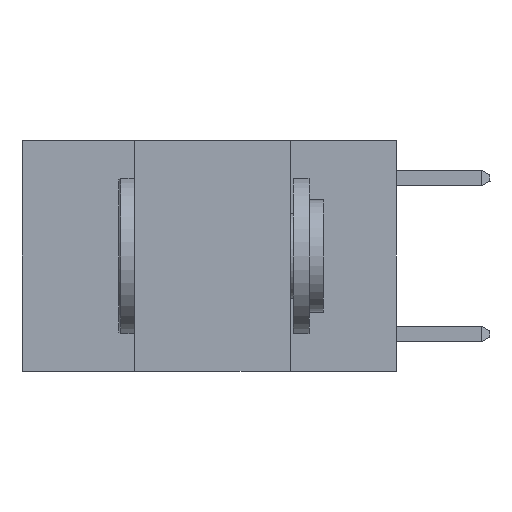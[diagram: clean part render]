
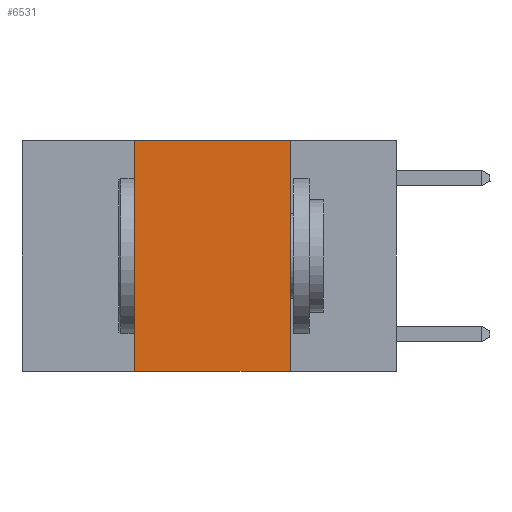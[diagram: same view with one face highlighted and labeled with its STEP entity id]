
A CAD part, left-side view. The second image highlights one B-rep face of the part: STEP entity #6531.
In plain terms, the highlighted planar face has unit normal (-1, 0, 0).
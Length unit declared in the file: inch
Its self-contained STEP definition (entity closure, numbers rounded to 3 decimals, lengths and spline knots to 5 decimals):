
#1452 = LINE ( 'NONE', #12778, #8683 ) ;
#1490 = LINE ( 'NONE', #7999, #16613 ) ;
#2187 = LINE ( 'NONE', #18214, #9373 ) ;
#4486 = EDGE_CURVE ( 'NONE', #6804, #16520, #1452, .T. ) ;
#4678 = VECTOR ( 'NONE', #15822, 39.37008 ) ;
#6480 = FACE_OUTER_BOUND ( 'NONE', #9676, .T. ) ;
#6512 = CARTESIAN_POINT ( 'NONE',  ( 0., 0.42, -0.37 ) ) ;
#6531 = ADVANCED_FACE ( 'NONE', ( #6480 ), #7337, .F. ) ;
#6561 = DIRECTION ( 'NONE',  ( 0., -1., 0. ) ) ;
#6804 = VERTEX_POINT ( 'NONE', #6512 ) ;
#7207 = ORIENTED_EDGE ( 'NONE', *, *, #15661, .F. ) ;
#7337 = PLANE ( 'NONE',  #16276 ) ;
#7359 = CARTESIAN_POINT ( 'NONE',  ( 0., 0.42, 0. ) ) ;
#7409 = ORIENTED_EDGE ( 'NONE', *, *, #14850, .F. ) ;
#7429 = ORIENTED_EDGE ( 'NONE', *, *, #16599, .F. ) ;
#7681 = ORIENTED_EDGE ( 'NONE', *, *, #4486, .T. ) ;
#7999 = CARTESIAN_POINT ( 'NONE',  ( 0., 0.6, 0. ) ) ;
#8031 = LINE ( 'NONE', #7359, #4678 ) ;
#8585 = DIRECTION ( 'NONE',  ( 0., 0., -1. ) ) ;
#8683 = VECTOR ( 'NONE', #15579, 39.37008 ) ;
#8747 = DIRECTION ( 'NONE',  ( 0., 0., -1. ) ) ;
#8867 = VERTEX_POINT ( 'NONE', #14411 ) ;
#9373 = VECTOR ( 'NONE', #8585, 39.37008 ) ;
#9676 = EDGE_LOOP ( 'NONE', ( #7207, #7409, #7429, #7681 ) ) ;
#10503 = CARTESIAN_POINT ( 'NONE',  ( 0., 0.17, -0.37 ) ) ;
#12778 = CARTESIAN_POINT ( 'NONE',  ( 0., 0.6, -0.37 ) ) ;
#13037 = CARTESIAN_POINT ( 'NONE',  ( 0., 0.6, 0. ) ) ;
#14411 = CARTESIAN_POINT ( 'NONE',  ( 0., 0.17, 0. ) ) ;
#14850 = EDGE_CURVE ( 'NONE', #17914, #8867, #1490, .T. ) ;
#15579 = DIRECTION ( 'NONE',  ( 0., -1., 0. ) ) ;
#15661 = EDGE_CURVE ( 'NONE', #8867, #16520, #2187, .T. ) ;
#15822 = DIRECTION ( 'NONE',  ( 0., 0., 1. ) ) ;
#16276 = AXIS2_PLACEMENT_3D ( 'NONE', #13037, #17110, #8747 ) ;
#16520 = VERTEX_POINT ( 'NONE', #10503 ) ;
#16599 = EDGE_CURVE ( 'NONE', #6804, #17914, #8031, .T. ) ;
#16613 = VECTOR ( 'NONE', #6561, 39.37008 ) ;
#17110 = DIRECTION ( 'NONE',  ( 1., 0., 0. ) ) ;
#17264 = CARTESIAN_POINT ( 'NONE',  ( 0., 0.42, 0. ) ) ;
#17914 = VERTEX_POINT ( 'NONE', #17264 ) ;
#18214 = CARTESIAN_POINT ( 'NONE',  ( 0., 0.17, 0. ) ) ;
